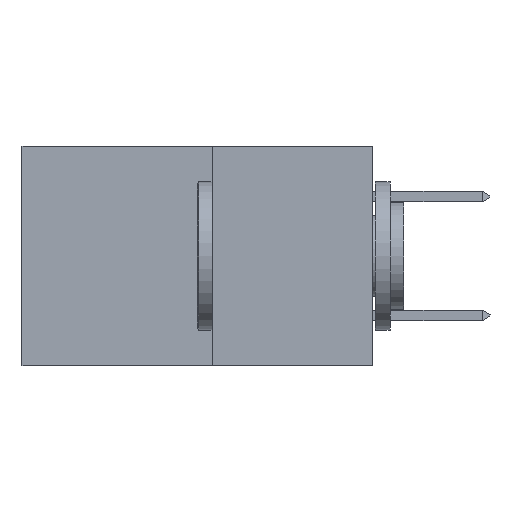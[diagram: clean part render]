
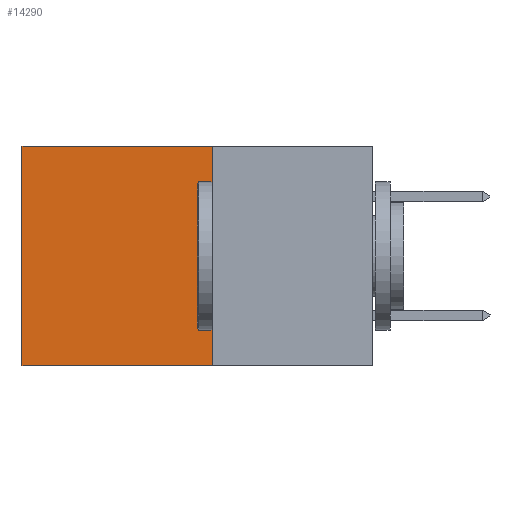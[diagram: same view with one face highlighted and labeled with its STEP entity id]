
A CAD part, left-side view. The second image highlights one B-rep face of the part: STEP entity #14290.
In plain terms, the highlighted planar face has unit normal (-1, 0, 0).
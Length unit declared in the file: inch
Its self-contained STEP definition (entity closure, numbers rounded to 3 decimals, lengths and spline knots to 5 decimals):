
#601 = CARTESIAN_POINT ( 'NONE',  ( 0.277, 0.27, 0. ) ) ;
#1321 = EDGE_CURVE ( 'NONE', #15389, #12424, #15742, .T. ) ;
#1330 = CARTESIAN_POINT ( 'NONE',  ( 0.277, 0.27, -0.37 ) ) ;
#2627 = DIRECTION ( 'NONE',  ( 0., 0., -1. ) ) ;
#3617 = DIRECTION ( 'NONE',  ( 0., 1., 0. ) ) ;
#3792 = AXIS2_PLACEMENT_3D ( 'NONE', #26386, #14292, #31195 ) ;
#4171 = PLANE ( 'NONE',  #3792 ) ;
#5486 = ORIENTED_EDGE ( 'NONE', *, *, #17085, .T. ) ;
#6542 = ORIENTED_EDGE ( 'NONE', *, *, #29193, .T. ) ;
#7467 = LINE ( 'NONE', #17574, #14143 ) ;
#9609 = DIRECTION ( 'NONE',  ( 0., 0., -1. ) ) ;
#9975 = CARTESIAN_POINT ( 'NONE',  ( 0.277, 0.27, -0.37 ) ) ;
#12424 = VERTEX_POINT ( 'NONE', #1330 ) ;
#13624 = CARTESIAN_POINT ( 'NONE',  ( 0.277, 0.27, -0.37 ) ) ;
#14143 = VECTOR ( 'NONE', #2627, 39.37008 ) ;
#14290 = ADVANCED_FACE ( 'NONE', ( #30818 ), #4171, .F. ) ;
#14292 = DIRECTION ( 'NONE',  ( 1., 0., 0. ) ) ;
#15389 = VERTEX_POINT ( 'NONE', #25385 ) ;
#15618 = DIRECTION ( 'NONE',  ( 0., 1., 0. ) ) ;
#15742 = LINE ( 'NONE', #9975, #27841 ) ;
#17085 = EDGE_CURVE ( 'NONE', #22238, #23305, #7467, .T. ) ;
#17574 = CARTESIAN_POINT ( 'NONE',  ( 0.277, 0.59, -0.37 ) ) ;
#18983 = CARTESIAN_POINT ( 'NONE',  ( 0.277, 0.59, -0.37 ) ) ;
#20670 = VECTOR ( 'NONE', #3617, 39.37008 ) ;
#22238 = VERTEX_POINT ( 'NONE', #22394 ) ;
#22394 = CARTESIAN_POINT ( 'NONE',  ( 0.277, 0.59, 0. ) ) ;
#22737 = LINE ( 'NONE', #601, #24235 ) ;
#22805 = ORIENTED_EDGE ( 'NONE', *, *, #23855, .F. ) ;
#23305 = VERTEX_POINT ( 'NONE', #18983 ) ;
#23855 = EDGE_CURVE ( 'NONE', #12424, #23305, #27831, .T. ) ;
#24235 = VECTOR ( 'NONE', #15618, 39.37008 ) ;
#25385 = CARTESIAN_POINT ( 'NONE',  ( 0.277, 0.27, 0. ) ) ;
#25760 = ORIENTED_EDGE ( 'NONE', *, *, #1321, .F. ) ;
#25865 = EDGE_LOOP ( 'NONE', ( #5486, #22805, #25760, #6542 ) ) ;
#26386 = CARTESIAN_POINT ( 'NONE',  ( 0.277, 0.27, -0.37 ) ) ;
#27831 = LINE ( 'NONE', #13624, #20670 ) ;
#27841 = VECTOR ( 'NONE', #9609, 39.37008 ) ;
#29193 = EDGE_CURVE ( 'NONE', #15389, #22238, #22737, .T. ) ;
#30818 = FACE_OUTER_BOUND ( 'NONE', #25865, .T. ) ;
#31195 = DIRECTION ( 'NONE',  ( 0., 0., -1. ) ) ;
